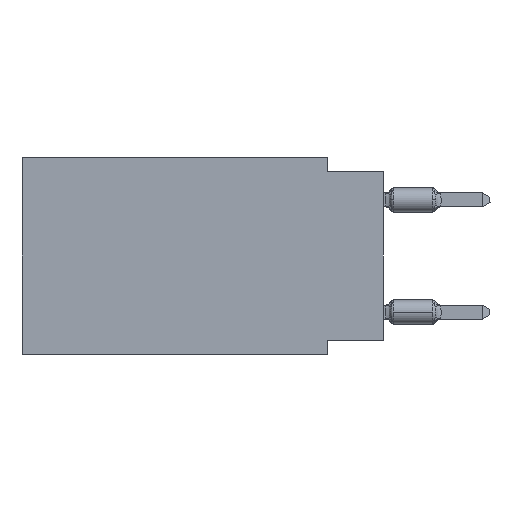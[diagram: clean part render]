
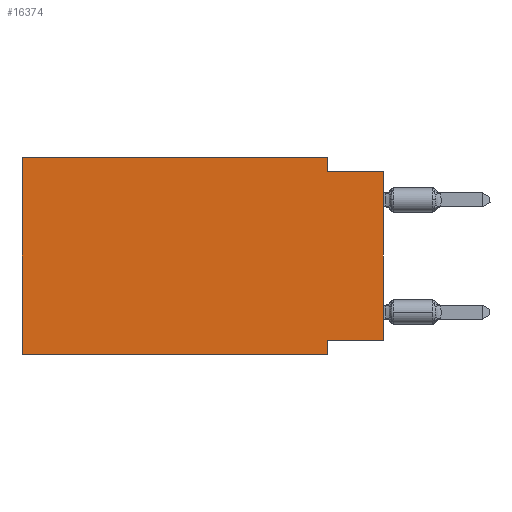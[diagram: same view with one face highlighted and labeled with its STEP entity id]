
A CAD part, left-side view. The second image highlights one B-rep face of the part: STEP entity #16374.
In plain terms, the highlighted planar face has unit normal (-1, 0, 0).
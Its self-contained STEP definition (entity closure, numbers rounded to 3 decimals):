
#208 = EDGE_CURVE ( 'NONE', #16445, #19571, #15130, .T. ) ;
#435 = CARTESIAN_POINT ( 'NONE',  ( 0., 2.54, 0. ) ) ;
#667 = VERTEX_POINT ( 'NONE', #1244 ) ;
#1163 = ORIENTED_EDGE ( 'NONE', *, *, #3686, .F. ) ;
#1244 = CARTESIAN_POINT ( 'NONE',  ( 0., 2.54, -8.255 ) ) ;
#1382 = EDGE_LOOP ( 'NONE', ( #11217, #10318, #1163, #3244, #6993, #12097, #5286, #10462 ) ) ;
#1593 = VERTEX_POINT ( 'NONE', #13065 ) ;
#2396 = CARTESIAN_POINT ( 'NONE',  ( 0., 2.54, -8.89 ) ) ;
#2860 = CARTESIAN_POINT ( 'NONE',  ( 0., 0., -0.635 ) ) ;
#3244 = ORIENTED_EDGE ( 'NONE', *, *, #208, .F. ) ;
#3686 = EDGE_CURVE ( 'NONE', #19571, #3896, #14286, .T. ) ;
#3896 = VERTEX_POINT ( 'NONE', #8431 ) ;
#4495 = DIRECTION ( 'NONE',  ( 0., -1., 0. ) ) ;
#5083 = VECTOR ( 'NONE', #4495, 1000. ) ;
#5087 = VERTEX_POINT ( 'NONE', #15318 ) ;
#5286 = ORIENTED_EDGE ( 'NONE', *, *, #6429, .F. ) ;
#5340 = EDGE_CURVE ( 'NONE', #1593, #5087, #8209, .T. ) ;
#5706 = FACE_OUTER_BOUND ( 'NONE', #1382, .T. ) ;
#6123 = CARTESIAN_POINT ( 'NONE',  ( 0., 2.54, 0. ) ) ;
#6371 = CARTESIAN_POINT ( 'NONE',  ( 0., 0., 0. ) ) ;
#6429 = EDGE_CURVE ( 'NONE', #667, #19877, #8980, .T. ) ;
#6993 = ORIENTED_EDGE ( 'NONE', *, *, #15625, .F. ) ;
#7248 = AXIS2_PLACEMENT_3D ( 'NONE', #15457, #7840, #17184 ) ;
#7298 = DIRECTION ( 'NONE',  ( 0., -1., 0. ) ) ;
#7315 = CARTESIAN_POINT ( 'NONE',  ( 0., 16.383, 0. ) ) ;
#7359 = VECTOR ( 'NONE', #16046, 1000. ) ;
#7371 = LINE ( 'NONE', #2860, #5083 ) ;
#7840 = DIRECTION ( 'NONE',  ( 1., 0., 0. ) ) ;
#8209 = LINE ( 'NONE', #6371, #16263 ) ;
#8431 = CARTESIAN_POINT ( 'NONE',  ( 0., 2.54, -0.635 ) ) ;
#8464 = EDGE_CURVE ( 'NONE', #17065, #19877, #17861, .T. ) ;
#8486 = EDGE_CURVE ( 'NONE', #1593, #667, #17765, .T. ) ;
#8777 = VECTOR ( 'NONE', #10062, 1000. ) ;
#8980 = LINE ( 'NONE', #13590, #10407 ) ;
#10062 = DIRECTION ( 'NONE',  ( 0., 1., 0. ) ) ;
#10318 = ORIENTED_EDGE ( 'NONE', *, *, #18940, .F. ) ;
#10369 = CARTESIAN_POINT ( 'NONE',  ( 0., 0., -8.255 ) ) ;
#10407 = VECTOR ( 'NONE', #11843, 1000. ) ;
#10462 = ORIENTED_EDGE ( 'NONE', *, *, #8486, .F. ) ;
#11103 = CARTESIAN_POINT ( 'NONE',  ( 0., 16.383, 0. ) ) ;
#11217 = ORIENTED_EDGE ( 'NONE', *, *, #5340, .T. ) ;
#11699 = CARTESIAN_POINT ( 'NONE',  ( 0., 16.383, -8.89 ) ) ;
#11843 = DIRECTION ( 'NONE',  ( 0., 0., -1. ) ) ;
#11943 = PLANE ( 'NONE',  #7248 ) ;
#12097 = ORIENTED_EDGE ( 'NONE', *, *, #8464, .T. ) ;
#13065 = CARTESIAN_POINT ( 'NONE',  ( 0., 0., -8.255 ) ) ;
#13590 = CARTESIAN_POINT ( 'NONE',  ( 0., 2.54, -8.89 ) ) ;
#13781 = VECTOR ( 'NONE', #15319, 1000. ) ;
#14286 = LINE ( 'NONE', #435, #7359 ) ;
#15130 = LINE ( 'NONE', #7315, #17355 ) ;
#15215 = LINE ( 'NONE', #19912, #13781 ) ;
#15223 = DIRECTION ( 'NONE',  ( 0., -1., 0. ) ) ;
#15318 = CARTESIAN_POINT ( 'NONE',  ( 0., 0., -0.635 ) ) ;
#15319 = DIRECTION ( 'NONE',  ( 0., 0., 1. ) ) ;
#15457 = CARTESIAN_POINT ( 'NONE',  ( 0., 16.383, 0. ) ) ;
#15625 = EDGE_CURVE ( 'NONE', #17065, #16445, #15215, .T. ) ;
#16046 = DIRECTION ( 'NONE',  ( 0., 0., -1. ) ) ;
#16263 = VECTOR ( 'NONE', #17650, 1000. ) ;
#16374 = ADVANCED_FACE ( 'NONE', ( #5706 ), #11943, .F. ) ;
#16445 = VERTEX_POINT ( 'NONE', #11103 ) ;
#17065 = VERTEX_POINT ( 'NONE', #18153 ) ;
#17184 = DIRECTION ( 'NONE',  ( 0., 0., -1. ) ) ;
#17306 = VECTOR ( 'NONE', #7298, 1000. ) ;
#17355 = VECTOR ( 'NONE', #15223, 1000. ) ;
#17650 = DIRECTION ( 'NONE',  ( 0., 0., 1. ) ) ;
#17765 = LINE ( 'NONE', #10369, #8777 ) ;
#17861 = LINE ( 'NONE', #11699, #17306 ) ;
#18153 = CARTESIAN_POINT ( 'NONE',  ( 0., 16.383, -8.89 ) ) ;
#18940 = EDGE_CURVE ( 'NONE', #3896, #5087, #7371, .T. ) ;
#19571 = VERTEX_POINT ( 'NONE', #6123 ) ;
#19877 = VERTEX_POINT ( 'NONE', #2396 ) ;
#19912 = CARTESIAN_POINT ( 'NONE',  ( 0., 16.383, 0. ) ) ;
